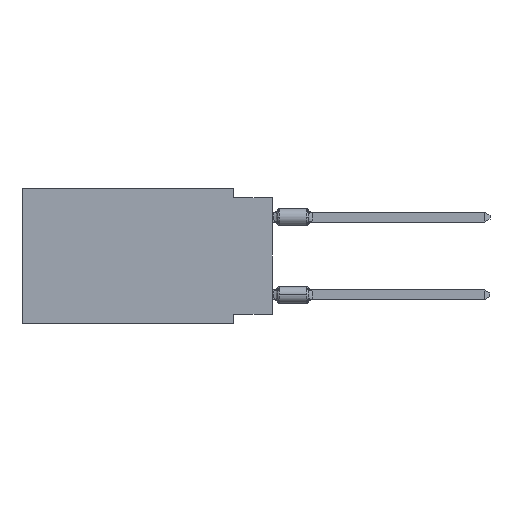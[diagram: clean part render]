
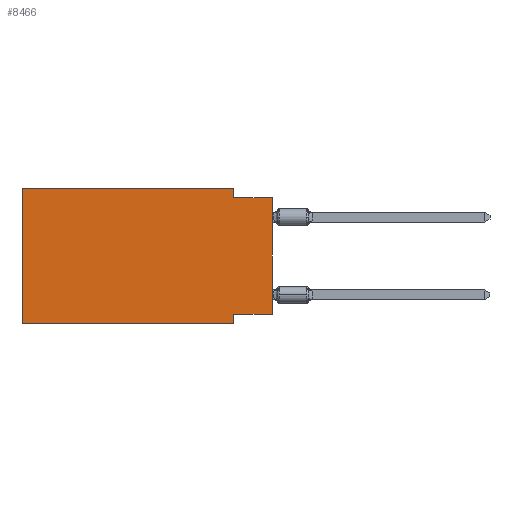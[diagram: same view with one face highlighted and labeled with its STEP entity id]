
A CAD part, left-side view. The second image highlights one B-rep face of the part: STEP entity #8466.
In plain terms, the highlighted planar face has unit normal (-1, 0, 0).
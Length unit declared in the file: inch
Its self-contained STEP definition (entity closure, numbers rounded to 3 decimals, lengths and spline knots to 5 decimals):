
#474 = VECTOR ( 'NONE', #13066, 39.37008 ) ;
#556 = DIRECTION ( 'NONE',  ( 0., -1., 0. ) ) ;
#938 = EDGE_CURVE ( 'NONE', #6295, #7505, #11621, .T. ) ;
#1351 = ORIENTED_EDGE ( 'NONE', *, *, #9618, .F. ) ;
#2125 = EDGE_CURVE ( 'NONE', #23043, #2647, #10383, .T. ) ;
#2647 = VERTEX_POINT ( 'NONE', #16197 ) ;
#2839 = CARTESIAN_POINT ( 'NONE',  ( 0., 0.645, 0. ) ) ;
#4461 = CARTESIAN_POINT ( 'NONE',  ( 0., 0., 0. ) ) ;
#4598 = ORIENTED_EDGE ( 'NONE', *, *, #11617, .T. ) ;
#4945 = PLANE ( 'NONE',  #10579 ) ;
#5657 = LINE ( 'NONE', #24649, #15451 ) ;
#5901 = CARTESIAN_POINT ( 'NONE',  ( 0., 0.1, 0. ) ) ;
#6119 = ORIENTED_EDGE ( 'NONE', *, *, #22916, .T. ) ;
#6295 = VERTEX_POINT ( 'NONE', #20386 ) ;
#6340 = DIRECTION ( 'NONE',  ( 0., 0., -1. ) ) ;
#6376 = CARTESIAN_POINT ( 'NONE',  ( 0., 0., -0.025 ) ) ;
#6506 = CARTESIAN_POINT ( 'NONE',  ( 0., 0., -0.325 ) ) ;
#7505 = VERTEX_POINT ( 'NONE', #21521 ) ;
#7558 = DIRECTION ( 'NONE',  ( 0., -1., 0. ) ) ;
#8466 = ADVANCED_FACE ( 'NONE', ( #19944 ), #4945, .F. ) ;
#8558 = LINE ( 'NONE', #10413, #17551 ) ;
#8746 = ORIENTED_EDGE ( 'NONE', *, *, #16180, .F. ) ;
#9420 = CARTESIAN_POINT ( 'NONE',  ( 0., 0.645, 0. ) ) ;
#9618 = EDGE_CURVE ( 'NONE', #16045, #19379, #23475, .T. ) ;
#10207 = DIRECTION ( 'NONE',  ( 1., 0., 0. ) ) ;
#10375 = VERTEX_POINT ( 'NONE', #15439 ) ;
#10383 = LINE ( 'NONE', #6506, #13711 ) ;
#10413 = CARTESIAN_POINT ( 'NONE',  ( 0., 0.645, 0. ) ) ;
#10579 = AXIS2_PLACEMENT_3D ( 'NONE', #2839, #10207, #6340 ) ;
#10735 = CARTESIAN_POINT ( 'NONE',  ( 0., 0., -0.025 ) ) ;
#10752 = VERTEX_POINT ( 'NONE', #5901 ) ;
#11569 = DIRECTION ( 'NONE',  ( 0., 0., 1. ) ) ;
#11617 = EDGE_CURVE ( 'NONE', #23043, #19379, #13948, .T. ) ;
#11621 = LINE ( 'NONE', #9420, #23083 ) ;
#12132 = CARTESIAN_POINT ( 'NONE',  ( 0., 0., -0.325 ) ) ;
#12291 = EDGE_CURVE ( 'NONE', #7505, #10752, #8558, .T. ) ;
#12797 = VECTOR ( 'NONE', #15670, 39.37008 ) ;
#13066 = DIRECTION ( 'NONE',  ( 0., 0., -1. ) ) ;
#13711 = VECTOR ( 'NONE', #19876, 39.37008 ) ;
#13741 = ORIENTED_EDGE ( 'NONE', *, *, #14845, .F. ) ;
#13948 = LINE ( 'NONE', #4461, #23035 ) ;
#14449 = ORIENTED_EDGE ( 'NONE', *, *, #2125, .F. ) ;
#14845 = EDGE_CURVE ( 'NONE', #2647, #10375, #16708, .T. ) ;
#15259 = DIRECTION ( 'NONE',  ( 0., 0., 1. ) ) ;
#15434 = CARTESIAN_POINT ( 'NONE',  ( 0., 0.1, 0. ) ) ;
#15439 = CARTESIAN_POINT ( 'NONE',  ( 0., 0.1, -0.35 ) ) ;
#15451 = VECTOR ( 'NONE', #7558, 39.37008 ) ;
#15670 = DIRECTION ( 'NONE',  ( 0., 0., -1. ) ) ;
#16045 = VERTEX_POINT ( 'NONE', #24675 ) ;
#16180 = EDGE_CURVE ( 'NONE', #10752, #16045, #19549, .T. ) ;
#16197 = CARTESIAN_POINT ( 'NONE',  ( 0., 0.1, -0.325 ) ) ;
#16205 = VECTOR ( 'NONE', #23846, 39.37008 ) ;
#16708 = LINE ( 'NONE', #24415, #474 ) ;
#16803 = ORIENTED_EDGE ( 'NONE', *, *, #938, .F. ) ;
#17551 = VECTOR ( 'NONE', #556, 39.37008 ) ;
#19075 = ORIENTED_EDGE ( 'NONE', *, *, #12291, .F. ) ;
#19379 = VERTEX_POINT ( 'NONE', #10735 ) ;
#19549 = LINE ( 'NONE', #15434, #12797 ) ;
#19876 = DIRECTION ( 'NONE',  ( 0., 1., 0. ) ) ;
#19944 = FACE_OUTER_BOUND ( 'NONE', #24198, .T. ) ;
#20386 = CARTESIAN_POINT ( 'NONE',  ( 0., 0.645, -0.35 ) ) ;
#21521 = CARTESIAN_POINT ( 'NONE',  ( 0., 0.645, 0. ) ) ;
#22916 = EDGE_CURVE ( 'NONE', #6295, #10375, #5657, .T. ) ;
#23035 = VECTOR ( 'NONE', #11569, 39.37008 ) ;
#23043 = VERTEX_POINT ( 'NONE', #12132 ) ;
#23083 = VECTOR ( 'NONE', #15259, 39.37008 ) ;
#23475 = LINE ( 'NONE', #6376, #16205 ) ;
#23846 = DIRECTION ( 'NONE',  ( 0., -1., 0. ) ) ;
#24198 = EDGE_LOOP ( 'NONE', ( #4598, #1351, #8746, #19075, #16803, #6119, #13741, #14449 ) ) ;
#24415 = CARTESIAN_POINT ( 'NONE',  ( 0., 0.1, -0.35 ) ) ;
#24649 = CARTESIAN_POINT ( 'NONE',  ( 0., 0.645, -0.35 ) ) ;
#24675 = CARTESIAN_POINT ( 'NONE',  ( 0., 0.1, -0.025 ) ) ;
